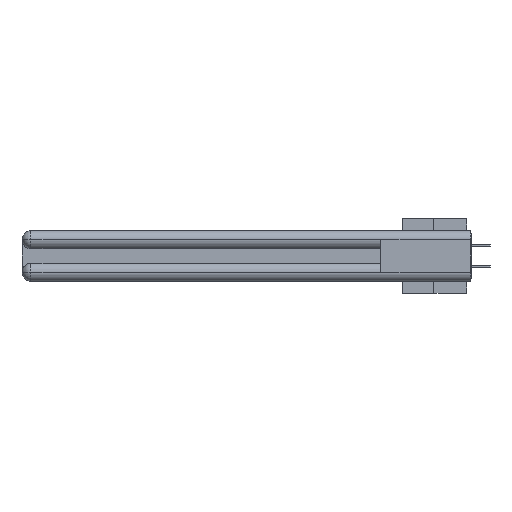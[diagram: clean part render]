
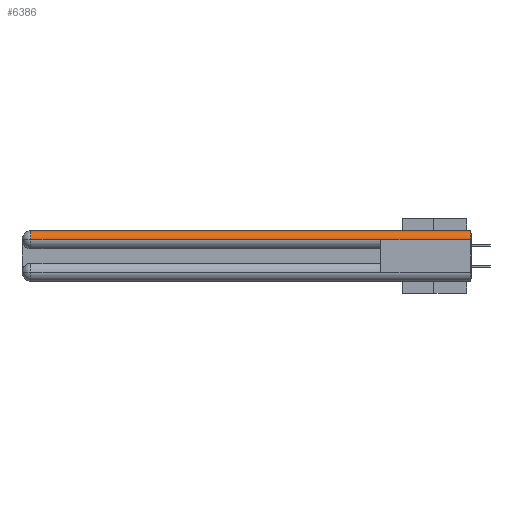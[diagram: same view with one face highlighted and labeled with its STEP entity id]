
A CAD part, left-side view. The second image highlights one B-rep face of the part: STEP entity #6386.
In plain terms, the highlighted cylindrical face has radius 1.562 mm (diameter 3.124 mm), a partial arc.
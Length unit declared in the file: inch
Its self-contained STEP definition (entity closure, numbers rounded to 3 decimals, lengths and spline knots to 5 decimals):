
#408 = EDGE_CURVE ( 'NONE', #31108, #27320, #18500, .T. ) ;
#829 = CARTESIAN_POINT ( 'NONE',  ( 0., 2.94, -0.0615 ) ) ;
#1153 = CARTESIAN_POINT ( 'NONE',  ( 0.0615, 0., 0. ) ) ;
#4809 = AXIS2_PLACEMENT_3D ( 'NONE', #34774, #29122, #9536 ) ;
#5006 = VECTOR ( 'NONE', #18279, 39.37008 ) ;
#5335 = AXIS2_PLACEMENT_3D ( 'NONE', #27068, #35341, #24023 ) ;
#5421 = CARTESIAN_POINT ( 'NONE',  ( 0., 3., -0.0615 ) ) ;
#5636 = ORIENTED_EDGE ( 'NONE', *, *, #30119, .F. ) ;
#6372 = CARTESIAN_POINT ( 'NONE',  ( 0., 0., -0.0615 ) ) ;
#6386 = ADVANCED_FACE ( 'NONE', ( #13241 ), #20261, .T. ) ;
#6572 = VECTOR ( 'NONE', #8309, 39.37008 ) ;
#7370 = EDGE_CURVE ( 'NONE', #28541, #9763, #31676, .T. ) ;
#7999 = DIRECTION ( 'NONE',  ( 0., -1., 0. ) ) ;
#8309 = DIRECTION ( 'NONE',  ( 0., 1., 0. ) ) ;
#8668 = CARTESIAN_POINT ( 'NONE',  ( 0., 3., -0.0615 ) ) ;
#9536 = DIRECTION ( 'NONE',  ( 0., 0., 1. ) ) ;
#9763 = VERTEX_POINT ( 'NONE', #829 ) ;
#12938 = EDGE_CURVE ( 'NONE', #9763, #27320, #33483, .T. ) ;
#13241 = FACE_OUTER_BOUND ( 'NONE', #36247, .T. ) ;
#16487 = LINE ( 'NONE', #1153, #5006 ) ;
#16800 = ORIENTED_EDGE ( 'NONE', *, *, #7370, .T. ) ;
#17021 = CARTESIAN_POINT ( 'NONE',  ( 0.0615, 0., 0. ) ) ;
#17902 = DIRECTION ( 'NONE',  ( 0., 1., 0. ) ) ;
#18279 = DIRECTION ( 'NONE',  ( 0., -1., 0. ) ) ;
#18500 = LINE ( 'NONE', #8668, #6572 ) ;
#20261 = CYLINDRICAL_SURFACE ( 'NONE', #30949, 0.0615 ) ;
#23717 = VERTEX_POINT ( 'NONE', #17021 ) ;
#24023 = DIRECTION ( 'NONE',  ( 1., 0., 0. ) ) ;
#26440 = VECTOR ( 'NONE', #7999, 39.37008 ) ;
#27068 = CARTESIAN_POINT ( 'NONE',  ( 0.0615, 0., -0.0615 ) ) ;
#27231 = CARTESIAN_POINT ( 'NONE',  ( 0., 0.6, -0.0615 ) ) ;
#27320 = VERTEX_POINT ( 'NONE', #27231 ) ;
#27902 = EDGE_CURVE ( 'NONE', #23717, #31108, #28861, .T. ) ;
#28541 = VERTEX_POINT ( 'NONE', #33008 ) ;
#28861 = CIRCLE ( 'NONE', #5335, 0.0615 ) ;
#29122 = DIRECTION ( 'NONE',  ( 0., -1., 0. ) ) ;
#29243 = DIRECTION ( 'NONE',  ( 0., 0., 1. ) ) ;
#30119 = EDGE_CURVE ( 'NONE', #28541, #23717, #16487, .T. ) ;
#30526 = ORIENTED_EDGE ( 'NONE', *, *, #27902, .F. ) ;
#30949 = AXIS2_PLACEMENT_3D ( 'NONE', #31813, #17902, #29243 ) ;
#31108 = VERTEX_POINT ( 'NONE', #6372 ) ;
#31262 = ORIENTED_EDGE ( 'NONE', *, *, #12938, .T. ) ;
#31676 = CIRCLE ( 'NONE', #4809, 0.0615 ) ;
#31813 = CARTESIAN_POINT ( 'NONE',  ( 0.0615, 0., -0.0615 ) ) ;
#33008 = CARTESIAN_POINT ( 'NONE',  ( 0.0615, 2.94, 0. ) ) ;
#33483 = LINE ( 'NONE', #5421, #26440 ) ;
#34774 = CARTESIAN_POINT ( 'NONE',  ( 0.0615, 2.94, -0.0615 ) ) ;
#35075 = ORIENTED_EDGE ( 'NONE', *, *, #408, .F. ) ;
#35341 = DIRECTION ( 'NONE',  ( 0., -1., 0. ) ) ;
#36247 = EDGE_LOOP ( 'NONE', ( #5636, #16800, #31262, #35075, #30526 ) ) ;
